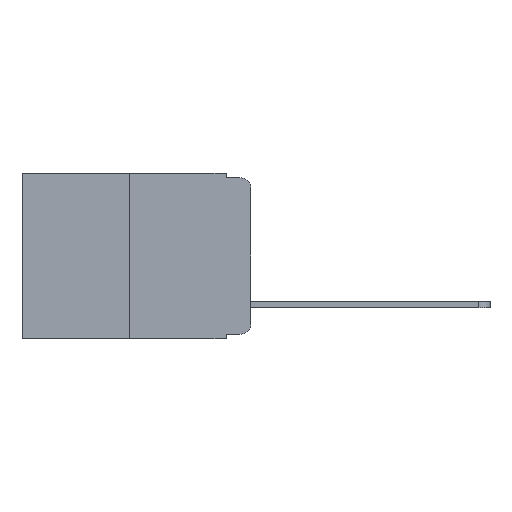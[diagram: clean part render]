
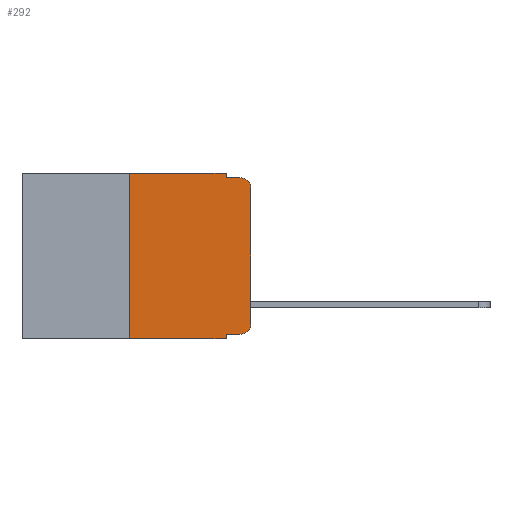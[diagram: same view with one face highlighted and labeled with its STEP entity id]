
A CAD part, left-side view. The second image highlights one B-rep face of the part: STEP entity #292.
In plain terms, the highlighted planar face has unit normal (-1, 0, 0).
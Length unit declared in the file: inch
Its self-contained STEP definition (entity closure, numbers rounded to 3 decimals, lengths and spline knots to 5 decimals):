
#79 = VECTOR ( 'NONE', #7043, 39.37008 ) ;
#155 = AXIS2_PLACEMENT_3D ( 'NONE', #14167, #3444, #15892 ) ;
#223 = VERTEX_POINT ( 'NONE', #1801 ) ;
#292 = ADVANCED_FACE ( 'NONE', ( #4772 ), #3980, .F. ) ;
#914 = DIRECTION ( 'NONE',  ( 0., 0., 1. ) ) ;
#1073 = CARTESIAN_POINT ( 'NONE',  ( 0., 0.25, 0. ) ) ;
#1103 = DIRECTION ( 'NONE',  ( 0., 0., -1. ) ) ;
#1603 = ORIENTED_EDGE ( 'NONE', *, *, #5134, .T. ) ;
#1719 = VERTEX_POINT ( 'NONE', #19951 ) ;
#1801 = CARTESIAN_POINT ( 'NONE',  ( 0., 0.02, -0.333 ) ) ;
#2293 = DIRECTION ( 'NONE',  ( 0., -1., 0. ) ) ;
#2800 = VERTEX_POINT ( 'NONE', #3695 ) ;
#2818 = CARTESIAN_POINT ( 'NONE',  ( 0., 0., -0.313 ) ) ;
#3120 = CIRCLE ( 'NONE', #155, 0.02 ) ;
#3273 = DIRECTION ( 'NONE',  ( 0., -1., 0. ) ) ;
#3444 = DIRECTION ( 'NONE',  ( -1., 0., 0. ) ) ;
#3695 = CARTESIAN_POINT ( 'NONE',  ( 0., 0.25, -0.343 ) ) ;
#3889 = ORIENTED_EDGE ( 'NONE', *, *, #5048, .T. ) ;
#3965 = EDGE_LOOP ( 'NONE', ( #3889, #22934, #8007, #14209, #11299, #11276, #8850, #5119, #9948, #1603 ) ) ;
#3980 = PLANE ( 'NONE',  #12058 ) ;
#4009 = CARTESIAN_POINT ( 'NONE',  ( 0., 0.473, 0. ) ) ;
#4041 = EDGE_CURVE ( 'NONE', #10543, #16994, #19235, .T. ) ;
#4369 = LINE ( 'NONE', #19168, #17280 ) ;
#4527 = EDGE_CURVE ( 'NONE', #2800, #8858, #9876, .T. ) ;
#4772 = FACE_OUTER_BOUND ( 'NONE', #3965, .T. ) ;
#4992 = LINE ( 'NONE', #19098, #79 ) ;
#5048 = EDGE_CURVE ( 'NONE', #12557, #1719, #10909, .T. ) ;
#5053 = EDGE_CURVE ( 'NONE', #1719, #5916, #14890, .T. ) ;
#5056 = EDGE_CURVE ( 'NONE', #15942, #5916, #19422, .T. ) ;
#5082 = EDGE_CURVE ( 'NONE', #16994, #15942, #4992, .T. ) ;
#5088 = EDGE_CURVE ( 'NONE', #2800, #10543, #22816, .T. ) ;
#5092 = EDGE_CURVE ( 'NONE', #8427, #8858, #9832, .T. ) ;
#5119 = ORIENTED_EDGE ( 'NONE', *, *, #5092, .F. ) ;
#5124 = EDGE_CURVE ( 'NONE', #8427, #223, #4369, .T. ) ;
#5134 = EDGE_CURVE ( 'NONE', #223, #12557, #3120, .T. ) ;
#5916 = VERTEX_POINT ( 'NONE', #5943 ) ;
#5943 = CARTESIAN_POINT ( 'NONE',  ( 0., 0.02, -0.01 ) ) ;
#6269 = CARTESIAN_POINT ( 'NONE',  ( 0., 0.473, 0. ) ) ;
#6970 = CARTESIAN_POINT ( 'NONE',  ( 0., 0.051, -0.01 ) ) ;
#7043 = DIRECTION ( 'NONE',  ( 0., 0., -1. ) ) ;
#8007 = ORIENTED_EDGE ( 'NONE', *, *, #5056, .F. ) ;
#8107 = CARTESIAN_POINT ( 'NONE',  ( 0., 0.473, -0.343 ) ) ;
#8427 = VERTEX_POINT ( 'NONE', #22374 ) ;
#8719 = CARTESIAN_POINT ( 'NONE',  ( 0., 0., 0. ) ) ;
#8797 = DIRECTION ( 'NONE',  ( -1., 0., 0. ) ) ;
#8850 = ORIENTED_EDGE ( 'NONE', *, *, #4527, .T. ) ;
#8858 = VERTEX_POINT ( 'NONE', #18522 ) ;
#8869 = CARTESIAN_POINT ( 'NONE',  ( 0., 0.051, 0. ) ) ;
#9291 = VECTOR ( 'NONE', #12333, 39.37008 ) ;
#9832 = LINE ( 'NONE', #8869, #22308 ) ;
#9876 = LINE ( 'NONE', #8107, #13327 ) ;
#9948 = ORIENTED_EDGE ( 'NONE', *, *, #5124, .T. ) ;
#10374 = VECTOR ( 'NONE', #914, 39.37008 ) ;
#10543 = VERTEX_POINT ( 'NONE', #1073 ) ;
#10618 = CARTESIAN_POINT ( 'NONE',  ( 0., 0.25, 0. ) ) ;
#10909 = LINE ( 'NONE', #8719, #10374 ) ;
#11276 = ORIENTED_EDGE ( 'NONE', *, *, #5088, .F. ) ;
#11299 = ORIENTED_EDGE ( 'NONE', *, *, #4041, .F. ) ;
#12058 = AXIS2_PLACEMENT_3D ( 'NONE', #4009, #20810, #20826 ) ;
#12333 = DIRECTION ( 'NONE',  ( 0., 0., 1. ) ) ;
#12557 = VERTEX_POINT ( 'NONE', #2818 ) ;
#13327 = VECTOR ( 'NONE', #15023, 39.37008 ) ;
#14167 = CARTESIAN_POINT ( 'NONE',  ( 0., 0.02, -0.313 ) ) ;
#14209 = ORIENTED_EDGE ( 'NONE', *, *, #5082, .F. ) ;
#14890 = CIRCLE ( 'NONE', #17766, 0.02 ) ;
#15023 = DIRECTION ( 'NONE',  ( 0., -1., 0. ) ) ;
#15892 = DIRECTION ( 'NONE',  ( 0., 0., -1. ) ) ;
#15942 = VERTEX_POINT ( 'NONE', #21807 ) ;
#16994 = VERTEX_POINT ( 'NONE', #22069 ) ;
#17280 = VECTOR ( 'NONE', #3273, 39.37008 ) ;
#17766 = AXIS2_PLACEMENT_3D ( 'NONE', #19016, #8797, #20726 ) ;
#18522 = CARTESIAN_POINT ( 'NONE',  ( 0., 0.051, -0.343 ) ) ;
#18679 = VECTOR ( 'NONE', #2293, 39.37008 ) ;
#18888 = VECTOR ( 'NONE', #22322, 39.37008 ) ;
#19016 = CARTESIAN_POINT ( 'NONE',  ( 0., 0.02, -0.03 ) ) ;
#19098 = CARTESIAN_POINT ( 'NONE',  ( 0., 0.051, 0. ) ) ;
#19168 = CARTESIAN_POINT ( 'NONE',  ( 0., 0.051, -0.333 ) ) ;
#19235 = LINE ( 'NONE', #6269, #18679 ) ;
#19422 = LINE ( 'NONE', #6970, #18888 ) ;
#19951 = CARTESIAN_POINT ( 'NONE',  ( 0., 0., -0.03 ) ) ;
#20726 = DIRECTION ( 'NONE',  ( 0., 0., -1. ) ) ;
#20810 = DIRECTION ( 'NONE',  ( 1., 0., 0. ) ) ;
#20826 = DIRECTION ( 'NONE',  ( 0., 0., -1. ) ) ;
#21807 = CARTESIAN_POINT ( 'NONE',  ( 0., 0.051, -0.01 ) ) ;
#22069 = CARTESIAN_POINT ( 'NONE',  ( 0., 0.051, 0. ) ) ;
#22308 = VECTOR ( 'NONE', #1103, 39.37008 ) ;
#22322 = DIRECTION ( 'NONE',  ( 0., -1., 0. ) ) ;
#22374 = CARTESIAN_POINT ( 'NONE',  ( 0., 0.051, -0.333 ) ) ;
#22816 = LINE ( 'NONE', #10618, #9291 ) ;
#22934 = ORIENTED_EDGE ( 'NONE', *, *, #5053, .T. ) ;
